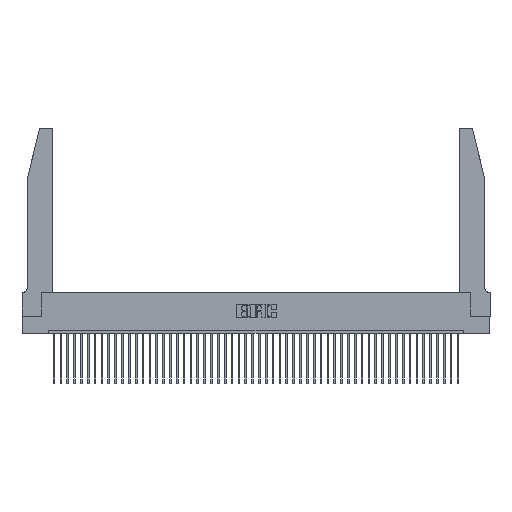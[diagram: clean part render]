
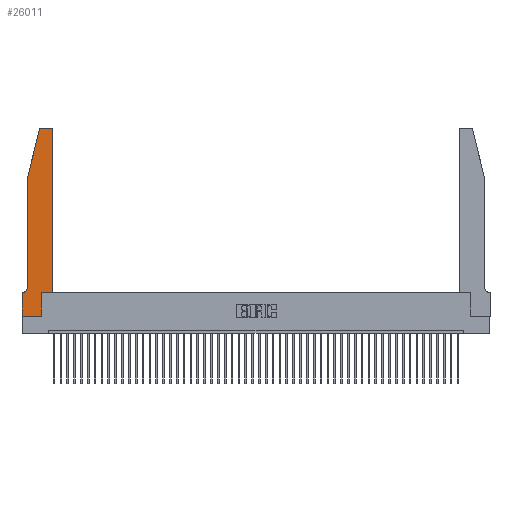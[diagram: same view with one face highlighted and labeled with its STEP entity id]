
A CAD part, top view. The second image highlights one B-rep face of the part: STEP entity #26011.
In plain terms, the highlighted planar face has unit normal (0, 0, 1).
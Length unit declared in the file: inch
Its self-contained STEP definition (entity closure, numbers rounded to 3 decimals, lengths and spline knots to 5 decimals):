
#655 = DIRECTION ( 'NONE',  ( 0., 0., 1. ) ) ;
#1053 = EDGE_CURVE ( 'NONE', #11999, #4075, #11187, .T. ) ;
#1351 = DIRECTION ( 'NONE',  ( 0., -1., 0. ) ) ;
#1451 = DIRECTION ( 'NONE',  ( 0., -1., 0. ) ) ;
#1838 = EDGE_CURVE ( 'NONE', #40430, #4620, #25490, .T. ) ;
#1995 = VERTEX_POINT ( 'NONE', #43916 ) ;
#2490 = VECTOR ( 'NONE', #45456, 39.37008 ) ;
#2726 = DIRECTION ( 'NONE',  ( 0., 0., -1. ) ) ;
#3002 = VERTEX_POINT ( 'NONE', #12089 ) ;
#3976 = EDGE_CURVE ( 'NONE', #35554, #42954, #26372, .T. ) ;
#4075 = VERTEX_POINT ( 'NONE', #31954 ) ;
#4206 = DIRECTION ( 'NONE',  ( 1., 0., 0. ) ) ;
#4291 = VECTOR ( 'NONE', #38352, 39.37008 ) ;
#4494 = DIRECTION ( 'NONE',  ( 1., 0., 0. ) ) ;
#4620 = VERTEX_POINT ( 'NONE', #10602 ) ;
#5046 = ORIENTED_EDGE ( 'NONE', *, *, #30972, .T. ) ;
#6965 = DIRECTION ( 'NONE',  ( 0., 1., 0. ) ) ;
#7215 = CARTESIAN_POINT ( 'NONE',  ( 0.4505, 2.72, 0.37 ) ) ;
#7907 = CARTESIAN_POINT ( 'NONE',  ( 0.4205, 2.72, 0.37 ) ) ;
#8023 = CARTESIAN_POINT ( 'NONE',  ( 0.0755, 2., 0.37 ) ) ;
#8562 = CARTESIAN_POINT ( 'NONE',  ( 0.2605, 2.75, 0.37 ) ) ;
#9070 = VECTOR ( 'NONE', #1351, 39.37008 ) ;
#9967 = EDGE_CURVE ( 'NONE', #32187, #12849, #39880, .T. ) ;
#10189 = VECTOR ( 'NONE', #1451, 39.37008 ) ;
#10194 = ORIENTED_EDGE ( 'NONE', *, *, #1838, .T. ) ;
#10602 = CARTESIAN_POINT ( 'NONE',  ( 0.25487, 2.72718, 0.37 ) ) ;
#11187 = CIRCLE ( 'NONE', #11327, 0.07 ) ;
#11327 = AXIS2_PLACEMENT_3D ( 'NONE', #36276, #2726, #22464 ) ;
#11421 = CARTESIAN_POINT ( 'NONE',  ( 0.284, 2.72, 0.37 ) ) ;
#11999 = VERTEX_POINT ( 'NONE', #13453 ) ;
#12089 = CARTESIAN_POINT ( 'NONE',  ( 0.4205, 2.75, 0.37 ) ) ;
#12337 = VECTOR ( 'NONE', #46405, 39.37008 ) ;
#12371 = CARTESIAN_POINT ( 'NONE',  ( 0.4505, 0.35, 0.37 ) ) ;
#12849 = VERTEX_POINT ( 'NONE', #7215 ) ;
#13453 = CARTESIAN_POINT ( 'NONE',  ( 0.0755, 0.42, 0.37 ) ) ;
#14680 = AXIS2_PLACEMENT_3D ( 'NONE', #7907, #22181, #4206 ) ;
#14974 = CARTESIAN_POINT ( 'NONE',  ( 0.0755, 0.35, 0.37 ) ) ;
#15937 = DIRECTION ( 'NONE',  ( -0.239, -0.971, 0. ) ) ;
#18473 = EDGE_CURVE ( 'NONE', #4620, #27027, #32553, .T. ) ;
#19489 = FACE_OUTER_BOUND ( 'NONE', #47359, .T. ) ;
#21130 = VECTOR ( 'NONE', #15937, 39.37008 ) ;
#21761 = CARTESIAN_POINT ( 'NONE',  ( 0., 0., 0.37 ) ) ;
#22000 = LINE ( 'NONE', #30854, #2490 ) ;
#22181 = DIRECTION ( 'NONE',  ( 0., 0., 1. ) ) ;
#22464 = DIRECTION ( 'NONE',  ( -1., 0., 0. ) ) ;
#22804 = LINE ( 'NONE', #27623, #10189 ) ;
#22930 = ORIENTED_EDGE ( 'NONE', *, *, #29434, .T. ) ;
#23361 = AXIS2_PLACEMENT_3D ( 'NONE', #11421, #655, #4494 ) ;
#23552 = ORIENTED_EDGE ( 'NONE', *, *, #18473, .T. ) ;
#23950 = DIRECTION ( 'NONE',  ( -1., 0., 0. ) ) ;
#24445 = CARTESIAN_POINT ( 'NONE',  ( 0.4505, 0.35, 0.37 ) ) ;
#24646 = ORIENTED_EDGE ( 'NONE', *, *, #24782, .T. ) ;
#24782 = EDGE_CURVE ( 'NONE', #12849, #3002, #40754, .T. ) ;
#25490 = CIRCLE ( 'NONE', #23361, 0.03 ) ;
#26011 = ADVANCED_FACE ( 'NONE', ( #19489 ), #27232, .T. ) ;
#26372 = LINE ( 'NONE', #29087, #38446 ) ;
#27027 = VERTEX_POINT ( 'NONE', #8023 ) ;
#27224 = EDGE_CURVE ( 'NONE', #27027, #11999, #22804, .T. ) ;
#27232 = PLANE ( 'NONE',  #33734 ) ;
#27377 = CARTESIAN_POINT ( 'NONE',  ( 0., 0.35, 0.37 ) ) ;
#27623 = CARTESIAN_POINT ( 'NONE',  ( 0.0755, 2., 0.37 ) ) ;
#27829 = VECTOR ( 'NONE', #23950, 39.37008 ) ;
#28038 = VECTOR ( 'NONE', #33530, 39.37008 ) ;
#29087 = CARTESIAN_POINT ( 'NONE',  ( 0.2865, 0.35, 0.37 ) ) ;
#29434 = EDGE_CURVE ( 'NONE', #3002, #40430, #30061, .T. ) ;
#30061 = LINE ( 'NONE', #8562, #27829 ) ;
#30854 = CARTESIAN_POINT ( 'NONE',  ( 0., 0., 0.37 ) ) ;
#30972 = EDGE_CURVE ( 'NONE', #1995, #33708, #43534, .T. ) ;
#31518 = ORIENTED_EDGE ( 'NONE', *, *, #1053, .T. ) ;
#31523 = DIRECTION ( 'NONE',  ( 1., 0., 0. ) ) ;
#31954 = CARTESIAN_POINT ( 'NONE',  ( 0.0055, 0.35, 0.37 ) ) ;
#32187 = VERTEX_POINT ( 'NONE', #32912 ) ;
#32553 = LINE ( 'NONE', #44785, #21130 ) ;
#32912 = CARTESIAN_POINT ( 'NONE',  ( 0.4505, 0.35, 0.37 ) ) ;
#33347 = CARTESIAN_POINT ( 'NONE',  ( 0., 0., 0.37 ) ) ;
#33530 = DIRECTION ( 'NONE',  ( -1., 0., 0. ) ) ;
#33708 = VERTEX_POINT ( 'NONE', #33347 ) ;
#33734 = AXIS2_PLACEMENT_3D ( 'NONE', #27377, #42087, #31523 ) ;
#34288 = ORIENTED_EDGE ( 'NONE', *, *, #35037, .T. ) ;
#34669 = ORIENTED_EDGE ( 'NONE', *, *, #27224, .T. ) ;
#35037 = EDGE_CURVE ( 'NONE', #4075, #1995, #47523, .T. ) ;
#35126 = CARTESIAN_POINT ( 'NONE',  ( 0.284, 2.75, 0.37 ) ) ;
#35554 = VERTEX_POINT ( 'NONE', #46711 ) ;
#36276 = CARTESIAN_POINT ( 'NONE',  ( 0.0055, 0.42, 0.37 ) ) ;
#36467 = LINE ( 'NONE', #12371, #4291 ) ;
#38352 = DIRECTION ( 'NONE',  ( 1., 0., 0. ) ) ;
#38446 = VECTOR ( 'NONE', #6965, 39.37008 ) ;
#39880 = LINE ( 'NONE', #24445, #12337 ) ;
#40074 = ORIENTED_EDGE ( 'NONE', *, *, #3976, .T. ) ;
#40430 = VERTEX_POINT ( 'NONE', #35126 ) ;
#40754 = CIRCLE ( 'NONE', #14680, 0.03 ) ;
#40808 = ORIENTED_EDGE ( 'NONE', *, *, #9967, .T. ) ;
#42087 = DIRECTION ( 'NONE',  ( 0., 0., 1. ) ) ;
#42954 = VERTEX_POINT ( 'NONE', #46754 ) ;
#43534 = LINE ( 'NONE', #21761, #9070 ) ;
#43916 = CARTESIAN_POINT ( 'NONE',  ( 0., 0.35, 0.37 ) ) ;
#44785 = CARTESIAN_POINT ( 'NONE',  ( 0.0755, 2., 0.37 ) ) ;
#45456 = DIRECTION ( 'NONE',  ( 1., 0., 0. ) ) ;
#45706 = ORIENTED_EDGE ( 'NONE', *, *, #45878, .T. ) ;
#45841 = ORIENTED_EDGE ( 'NONE', *, *, #47004, .T. ) ;
#45878 = EDGE_CURVE ( 'NONE', #42954, #32187, #36467, .T. ) ;
#46405 = DIRECTION ( 'NONE',  ( 0., 1., 0. ) ) ;
#46711 = CARTESIAN_POINT ( 'NONE',  ( 0.2865, 0., 0.37 ) ) ;
#46754 = CARTESIAN_POINT ( 'NONE',  ( 0.2865, 0.35, 0.37 ) ) ;
#47004 = EDGE_CURVE ( 'NONE', #33708, #35554, #22000, .T. ) ;
#47359 = EDGE_LOOP ( 'NONE', ( #22930, #10194, #23552, #34669, #31518, #34288, #5046, #45841, #40074, #45706, #40808, #24646 ) ) ;
#47523 = LINE ( 'NONE', #14974, #28038 ) ;
